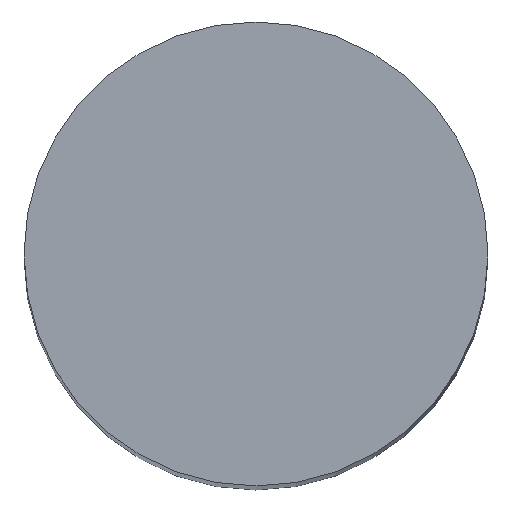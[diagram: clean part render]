
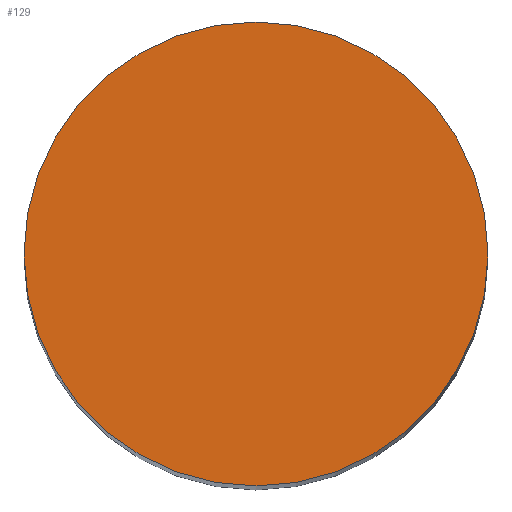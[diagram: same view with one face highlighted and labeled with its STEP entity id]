
A CAD part, top view. The second image highlights one B-rep face of the part: STEP entity #129.
In plain terms, the highlighted planar face has unit normal (0, 0, 1).
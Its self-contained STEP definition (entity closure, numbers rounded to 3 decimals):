
#8 = DIRECTION ( 'NONE',  ( 1., 0., 0. ) ) ;
#10 = EDGE_LOOP ( 'NONE', ( #128, #125 ) ) ;
#16 = PLANE ( 'NONE',  #63 ) ;
#26 = DIRECTION ( 'NONE',  ( 0., 0., 1. ) ) ;
#31 = CIRCLE ( 'NONE', #107, 2.5 ) ;
#32 = VERTEX_POINT ( 'NONE', #52 ) ;
#33 = FACE_OUTER_BOUND ( 'NONE', #10, .T. ) ;
#34 = CIRCLE ( 'NONE', #114, 2.5 ) ;
#37 = DIRECTION ( 'NONE',  ( 0., 0., 1. ) ) ;
#52 = CARTESIAN_POINT ( 'NONE',  ( 2.5, 0., 12.5 ) ) ;
#54 = DIRECTION ( 'NONE',  ( 0., 0., 1. ) ) ;
#63 = AXIS2_PLACEMENT_3D ( 'NONE', #92, #26, #110 ) ;
#67 = VERTEX_POINT ( 'NONE', #138 ) ;
#86 = EDGE_CURVE ( 'NONE', #32, #67, #31, .T. ) ;
#92 = CARTESIAN_POINT ( 'NONE',  ( 0., 0., 12.5 ) ) ;
#105 = CARTESIAN_POINT ( 'NONE',  ( 0., 0., 12.5 ) ) ;
#107 = AXIS2_PLACEMENT_3D ( 'NONE', #133, #54, #137 ) ;
#109 = EDGE_CURVE ( 'NONE', #67, #32, #34, .T. ) ;
#110 = DIRECTION ( 'NONE',  ( 1., 0., 0. ) ) ;
#114 = AXIS2_PLACEMENT_3D ( 'NONE', #105, #37, #8 ) ;
#125 = ORIENTED_EDGE ( 'NONE', *, *, #86, .T. ) ;
#128 = ORIENTED_EDGE ( 'NONE', *, *, #109, .T. ) ;
#129 = ADVANCED_FACE ( 'NONE', ( #33 ), #16, .T. ) ;
#133 = CARTESIAN_POINT ( 'NONE',  ( 0., 0., 12.5 ) ) ;
#137 = DIRECTION ( 'NONE',  ( 1., 0., 0. ) ) ;
#138 = CARTESIAN_POINT ( 'NONE',  ( -2.5, 0., 12.5 ) ) ;
